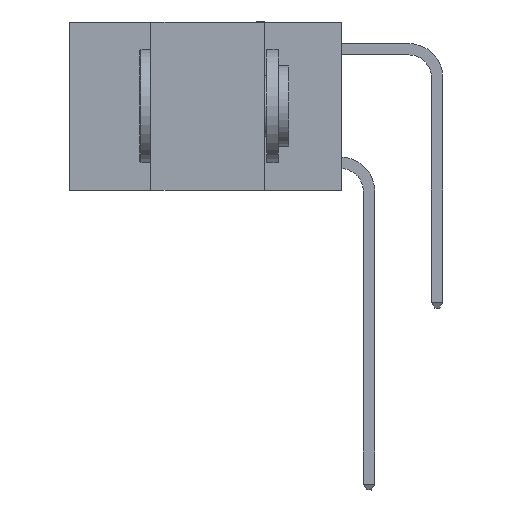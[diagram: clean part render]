
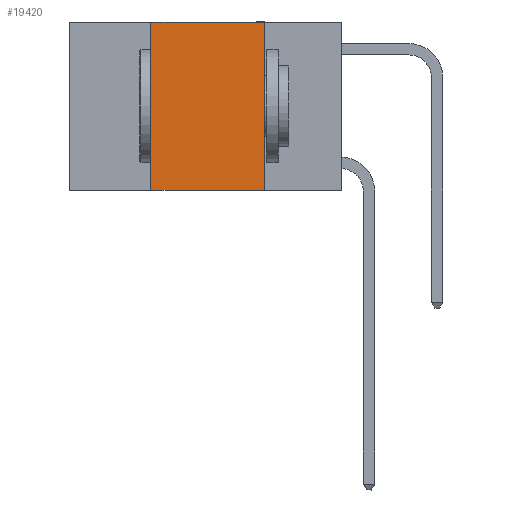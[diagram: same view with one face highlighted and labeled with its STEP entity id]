
A CAD part, left-side view. The second image highlights one B-rep face of the part: STEP entity #19420.
In plain terms, the highlighted planar face has unit normal (-1, 0, 0).
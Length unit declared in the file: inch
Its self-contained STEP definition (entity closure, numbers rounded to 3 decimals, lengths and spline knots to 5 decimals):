
#1479 = VECTOR ( 'NONE', #18023, 39.37008 ) ;
#2625 = CARTESIAN_POINT ( 'NONE',  ( 0., 0.17, 0. ) ) ;
#5341 = CARTESIAN_POINT ( 'NONE',  ( 0., 0.17, -0.37 ) ) ;
#5396 = VERTEX_POINT ( 'NONE', #2625 ) ;
#7633 = LINE ( 'NONE', #22171, #21417 ) ;
#7906 = DIRECTION ( 'NONE',  ( 0., -1., 0. ) ) ;
#8735 = FACE_OUTER_BOUND ( 'NONE', #25636, .T. ) ;
#8863 = DIRECTION ( 'NONE',  ( 0., 0., -1. ) ) ;
#8982 = EDGE_CURVE ( 'NONE', #5396, #18055, #17383, .T. ) ;
#9181 = ORIENTED_EDGE ( 'NONE', *, *, #25527, .F. ) ;
#9362 = CARTESIAN_POINT ( 'NONE',  ( 0., 0.6, 0. ) ) ;
#9387 = DIRECTION ( 'NONE',  ( 0., 0., 1. ) ) ;
#9414 = ORIENTED_EDGE ( 'NONE', *, *, #16047, .T. ) ;
#9551 = VERTEX_POINT ( 'NONE', #23291 ) ;
#9930 = ORIENTED_EDGE ( 'NONE', *, *, #23110, .F. ) ;
#11380 = LINE ( 'NONE', #9362, #1479 ) ;
#13031 = VECTOR ( 'NONE', #9387, 39.37008 ) ;
#15402 = DIRECTION ( 'NONE',  ( 1., 0., 0. ) ) ;
#16047 = EDGE_CURVE ( 'NONE', #9551, #18055, #7633, .T. ) ;
#16121 = ORIENTED_EDGE ( 'NONE', *, *, #8982, .F. ) ;
#16282 = CARTESIAN_POINT ( 'NONE',  ( 0., 0.42, 0. ) ) ;
#17383 = LINE ( 'NONE', #25089, #24310 ) ;
#17529 = LINE ( 'NONE', #24029, #13031 ) ;
#18023 = DIRECTION ( 'NONE',  ( 0., -1., 0. ) ) ;
#18055 = VERTEX_POINT ( 'NONE', #5341 ) ;
#18089 = AXIS2_PLACEMENT_3D ( 'NONE', #25508, #15402, #8863 ) ;
#19420 = ADVANCED_FACE ( 'NONE', ( #8735 ), #21127, .F. ) ;
#21127 = PLANE ( 'NONE',  #18089 ) ;
#21417 = VECTOR ( 'NONE', #7906, 39.37008 ) ;
#22171 = CARTESIAN_POINT ( 'NONE',  ( 0., 0.6, -0.37 ) ) ;
#23110 = EDGE_CURVE ( 'NONE', #23296, #5396, #11380, .T. ) ;
#23291 = CARTESIAN_POINT ( 'NONE',  ( 0., 0.42, -0.37 ) ) ;
#23296 = VERTEX_POINT ( 'NONE', #16282 ) ;
#24029 = CARTESIAN_POINT ( 'NONE',  ( 0., 0.42, 0. ) ) ;
#24310 = VECTOR ( 'NONE', #25476, 39.37008 ) ;
#25089 = CARTESIAN_POINT ( 'NONE',  ( 0., 0.17, 0. ) ) ;
#25476 = DIRECTION ( 'NONE',  ( 0., 0., -1. ) ) ;
#25508 = CARTESIAN_POINT ( 'NONE',  ( 0., 0.6, 0. ) ) ;
#25527 = EDGE_CURVE ( 'NONE', #9551, #23296, #17529, .T. ) ;
#25636 = EDGE_LOOP ( 'NONE', ( #16121, #9930, #9181, #9414 ) ) ;
